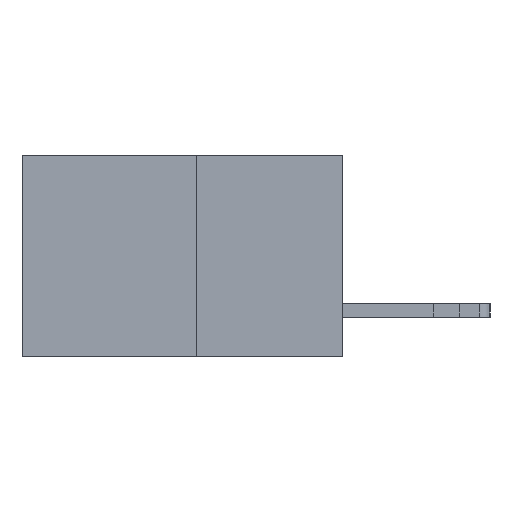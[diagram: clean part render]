
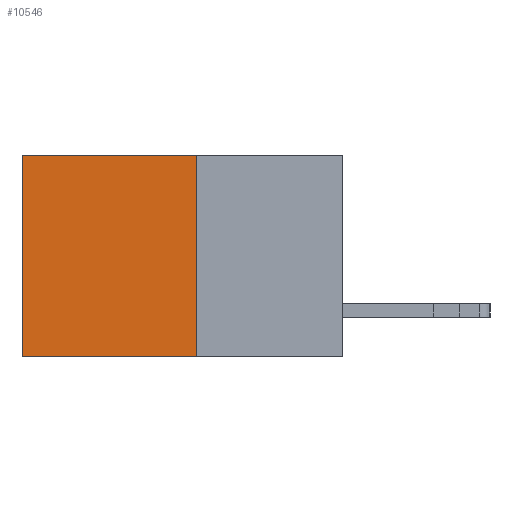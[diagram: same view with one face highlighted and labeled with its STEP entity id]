
A CAD part, left-side view. The second image highlights one B-rep face of the part: STEP entity #10546.
In plain terms, the highlighted planar face has unit normal (-1, 0, 0).
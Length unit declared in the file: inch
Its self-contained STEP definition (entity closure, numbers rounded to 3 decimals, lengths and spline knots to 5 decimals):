
#6 = DIRECTION ( 'NONE',  ( 0., 1., 0. ) ) ;
#203 = LINE ( 'NONE', #3618, #560 ) ;
#318 = VECTOR ( 'NONE', #6, 39.37008 ) ;
#560 = VECTOR ( 'NONE', #11112, 39.37008 ) ;
#1402 = CARTESIAN_POINT ( 'NONE',  ( 0.277, 0.27, -0.37 ) ) ;
#1943 = DIRECTION ( 'NONE',  ( 1., 0., 0. ) ) ;
#2489 = CARTESIAN_POINT ( 'NONE',  ( 0.277, 0.59, 0. ) ) ;
#2901 = ORIENTED_EDGE ( 'NONE', *, *, #13818, .T. ) ;
#2911 = ORIENTED_EDGE ( 'NONE', *, *, #13453, .F. ) ;
#3263 = EDGE_LOOP ( 'NONE', ( #13646, #6876, #2911, #2901 ) ) ;
#3560 = DIRECTION ( 'NONE',  ( 0., 0., -1. ) ) ;
#3572 = CARTESIAN_POINT ( 'NONE',  ( 0.277, 0.59, -0.37 ) ) ;
#3618 = CARTESIAN_POINT ( 'NONE',  ( 0.277, 0.27, 0. ) ) ;
#5094 = VECTOR ( 'NONE', #8865, 39.37008 ) ;
#5874 = VERTEX_POINT ( 'NONE', #1402 ) ;
#6270 = LINE ( 'NONE', #3572, #11917 ) ;
#6562 = EDGE_CURVE ( 'NONE', #11743, #13556, #6270, .T. ) ;
#6565 = CARTESIAN_POINT ( 'NONE',  ( 0.277, 0.27, 0. ) ) ;
#6876 = ORIENTED_EDGE ( 'NONE', *, *, #8695, .F. ) ;
#7112 = VERTEX_POINT ( 'NONE', #6565 ) ;
#7885 = LINE ( 'NONE', #12041, #5094 ) ;
#8409 = PLANE ( 'NONE',  #9762 ) ;
#8687 = CARTESIAN_POINT ( 'NONE',  ( 0.277, 0.27, -0.37 ) ) ;
#8695 = EDGE_CURVE ( 'NONE', #5874, #13556, #9023, .T. ) ;
#8865 = DIRECTION ( 'NONE',  ( 0., 0., -1. ) ) ;
#9023 = LINE ( 'NONE', #8687, #318 ) ;
#9503 = DIRECTION ( 'NONE',  ( 0., 0., -1. ) ) ;
#9762 = AXIS2_PLACEMENT_3D ( 'NONE', #13643, #1943, #9503 ) ;
#10546 = ADVANCED_FACE ( 'NONE', ( #10865 ), #8409, .F. ) ;
#10865 = FACE_OUTER_BOUND ( 'NONE', #3263, .T. ) ;
#11112 = DIRECTION ( 'NONE',  ( 0., 1., 0. ) ) ;
#11743 = VERTEX_POINT ( 'NONE', #2489 ) ;
#11917 = VECTOR ( 'NONE', #3560, 39.37008 ) ;
#12041 = CARTESIAN_POINT ( 'NONE',  ( 0.277, 0.27, -0.37 ) ) ;
#12267 = CARTESIAN_POINT ( 'NONE',  ( 0.277, 0.59, -0.37 ) ) ;
#13453 = EDGE_CURVE ( 'NONE', #7112, #5874, #7885, .T. ) ;
#13556 = VERTEX_POINT ( 'NONE', #12267 ) ;
#13643 = CARTESIAN_POINT ( 'NONE',  ( 0.277, 0.27, -0.37 ) ) ;
#13646 = ORIENTED_EDGE ( 'NONE', *, *, #6562, .T. ) ;
#13818 = EDGE_CURVE ( 'NONE', #7112, #11743, #203, .T. ) ;
